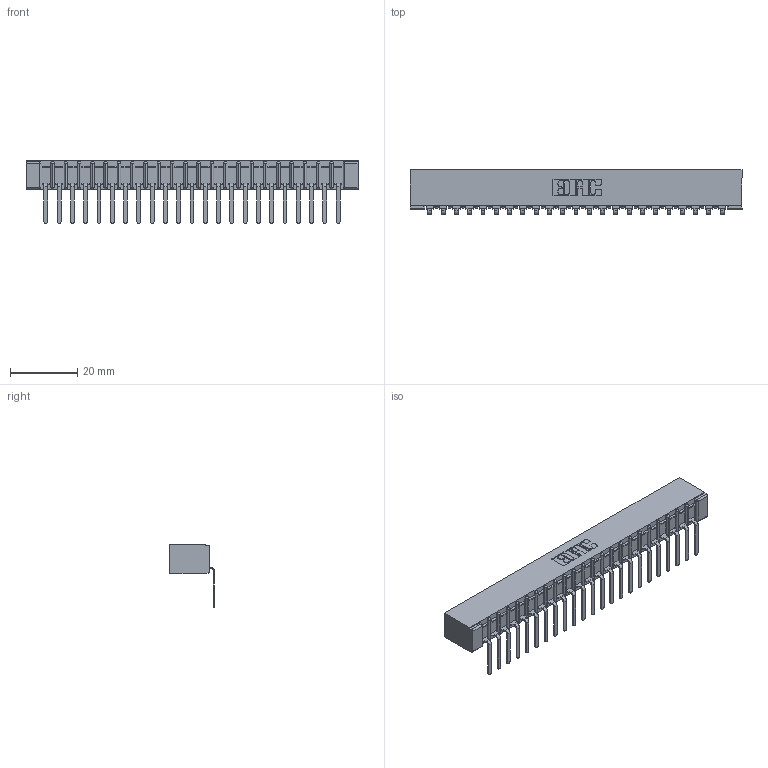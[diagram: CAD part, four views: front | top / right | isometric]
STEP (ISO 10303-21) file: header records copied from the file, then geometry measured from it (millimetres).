
FILE_DESCRIPTION (( 'STEP AP203' ), '1' );
FILE_NAME ('307-023-457-101.STEP', '2020-09-27T09:33:57', ( '' ), ( '' ), 'SwSTEP 2.0', 'SolidWorks 2020', '' );
FILE_SCHEMA (( 'CONFIG_CONTROL_DESIGN' ));
Length unit declared in the file: inch
Products named in the file (3): 307 Part_No Mounting Lugs; 307-290-002_557; 307-023-457-101
Assembly tree (24 placements, depth 2):
  307-023-457-101
    307 Part_No Mounting Lugs
    307-290-002_557  x23
Bounding box: 99.01 x 13.32 x 18.67 mm (x, y, z)
Volume: 6841.3 mm3; surface area: 13385.3 mm2
Topology: 24 solids, 24 shells, 1928 faces, 5911 edges, 3874 vertices
Faces by surface type: plane 1147, cylinder 733, sphere 48
Entity records: 22636 total; most frequent: CARTESIAN_POINT 3816, ORIENTED_EDGE 3806, DIRECTION 3715, EDGE_CURVE 1903, VECTOR 1449, LINE 1449, VERTEX_POINT 1234, AXIS2_PLACEMENT_3D 1133
